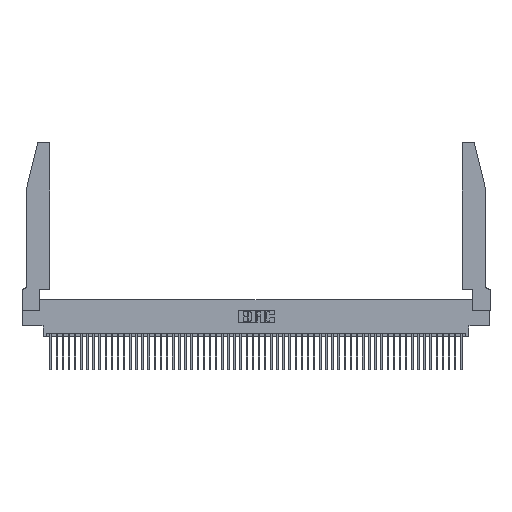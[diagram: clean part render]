
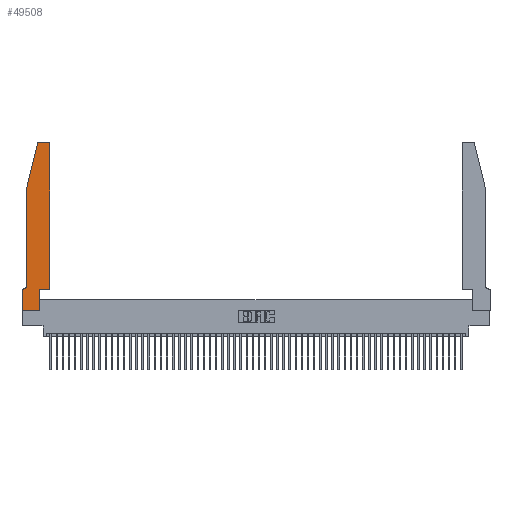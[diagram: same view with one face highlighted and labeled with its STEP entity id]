
A CAD part, top view. The second image highlights one B-rep face of the part: STEP entity #49508.
In plain terms, the highlighted planar face has unit normal (0, 0, 1).
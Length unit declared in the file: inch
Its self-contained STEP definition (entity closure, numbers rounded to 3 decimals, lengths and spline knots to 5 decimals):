
#418 = DIRECTION ( 'NONE',  ( 1., 0., 0. ) ) ;
#775 = EDGE_CURVE ( 'NONE', #7307, #12237, #3849, .T. ) ;
#871 = AXIS2_PLACEMENT_3D ( 'NONE', #14094, #43583, #18420 ) ;
#1311 = DIRECTION ( 'NONE',  ( 1., 0., 0. ) ) ;
#1388 = EDGE_CURVE ( 'NONE', #29535, #44781, #18639, .T. ) ;
#1393 = ORIENTED_EDGE ( 'NONE', *, *, #41156, .T. ) ;
#1676 = CARTESIAN_POINT ( 'NONE',  ( 0.4205, 2.75, 0.37 ) ) ;
#2209 = CARTESIAN_POINT ( 'NONE',  ( 0.25487, 2.72718, 0.37 ) ) ;
#3660 = CARTESIAN_POINT ( 'NONE',  ( 0.0755, 2., 0.37 ) ) ;
#3849 = LINE ( 'NONE', #41785, #36506 ) ;
#4893 = CARTESIAN_POINT ( 'NONE',  ( 0.2605, 2.75, 0.37 ) ) ;
#6025 = FACE_OUTER_BOUND ( 'NONE', #29176, .T. ) ;
#6207 = CARTESIAN_POINT ( 'NONE',  ( 0.4505, 0.35, 0.37 ) ) ;
#6626 = VERTEX_POINT ( 'NONE', #47167 ) ;
#6795 = ORIENTED_EDGE ( 'NONE', *, *, #48943, .T. ) ;
#7307 = VERTEX_POINT ( 'NONE', #44047 ) ;
#7408 = ORIENTED_EDGE ( 'NONE', *, *, #50088, .T. ) ;
#8753 = DIRECTION ( 'NONE',  ( -1., 0., 0. ) ) ;
#8770 = DIRECTION ( 'NONE',  ( 0., -1., 0. ) ) ;
#10470 = EDGE_CURVE ( 'NONE', #6626, #29535, #52792, .T. ) ;
#12237 = VERTEX_POINT ( 'NONE', #25831 ) ;
#12393 = VERTEX_POINT ( 'NONE', #30925 ) ;
#12711 = DIRECTION ( 'NONE',  ( 1., 0., 0. ) ) ;
#13014 = DIRECTION ( 'NONE',  ( -0.239, -0.971, 0. ) ) ;
#14094 = CARTESIAN_POINT ( 'NONE',  ( 0., 0.35, 0.37 ) ) ;
#14241 = ORIENTED_EDGE ( 'NONE', *, *, #775, .T. ) ;
#14365 = LINE ( 'NONE', #3660, #27088 ) ;
#14387 = LINE ( 'NONE', #29685, #36883 ) ;
#14700 = EDGE_CURVE ( 'NONE', #30006, #12393, #19690, .T. ) ;
#15366 = EDGE_CURVE ( 'NONE', #50289, #6626, #39972, .T. ) ;
#16240 = ORIENTED_EDGE ( 'NONE', *, *, #10470, .T. ) ;
#16377 = VERTEX_POINT ( 'NONE', #40725 ) ;
#17351 = CARTESIAN_POINT ( 'NONE',  ( 0.0755, 2., 0.37 ) ) ;
#17353 = CARTESIAN_POINT ( 'NONE',  ( 0.284, 2.75, 0.37 ) ) ;
#17538 = ORIENTED_EDGE ( 'NONE', *, *, #36465, .T. ) ;
#17938 = DIRECTION ( 'NONE',  ( -1., 0., 0. ) ) ;
#18100 = DIRECTION ( 'NONE',  ( 0., 1., 0. ) ) ;
#18420 = DIRECTION ( 'NONE',  ( 1., 0., 0. ) ) ;
#18639 = LINE ( 'NONE', #42083, #39715 ) ;
#19247 = CARTESIAN_POINT ( 'NONE',  ( 0., 0.35, 0.37 ) ) ;
#19675 = CIRCLE ( 'NONE', #27865, 0.03 ) ;
#19690 = LINE ( 'NONE', #17351, #28341 ) ;
#20626 = VERTEX_POINT ( 'NONE', #27876 ) ;
#23301 = CARTESIAN_POINT ( 'NONE',  ( 0., 0., 0.37 ) ) ;
#23875 = AXIS2_PLACEMENT_3D ( 'NONE', #50057, #25128, #54275 ) ;
#24315 = VECTOR ( 'NONE', #31812, 39.37008 ) ;
#25128 = DIRECTION ( 'NONE',  ( 0., 0., -1. ) ) ;
#25769 = AXIS2_PLACEMENT_3D ( 'NONE', #51171, #26213, #418 ) ;
#25831 = CARTESIAN_POINT ( 'NONE',  ( 0.4505, 0.35, 0.37 ) ) ;
#25879 = CARTESIAN_POINT ( 'NONE',  ( 0.0755, 0.35, 0.37 ) ) ;
#26213 = DIRECTION ( 'NONE',  ( 0., 0., 1. ) ) ;
#26536 = VECTOR ( 'NONE', #17938, 39.37008 ) ;
#27079 = DIRECTION ( 'NONE',  ( 0., 0., 1. ) ) ;
#27088 = VECTOR ( 'NONE', #8770, 39.37008 ) ;
#27865 = AXIS2_PLACEMENT_3D ( 'NONE', #52033, #27079, #1311 ) ;
#27876 = CARTESIAN_POINT ( 'NONE',  ( 0.4505, 2.72, 0.37 ) ) ;
#28341 = VECTOR ( 'NONE', #13014, 39.37008 ) ;
#29176 = EDGE_LOOP ( 'NONE', ( #17538, #7408, #34075, #32137, #33447, #16240, #31519, #53668, #1393, #14241, #6795, #33509 ) ) ;
#29295 = VECTOR ( 'NONE', #18100, 39.37008 ) ;
#29402 = EDGE_CURVE ( 'NONE', #20626, #43248, #19675, .T. ) ;
#29535 = VERTEX_POINT ( 'NONE', #19247 ) ;
#29685 = CARTESIAN_POINT ( 'NONE',  ( 0., 0., 0.37 ) ) ;
#30006 = VERTEX_POINT ( 'NONE', #2209 ) ;
#30714 = CARTESIAN_POINT ( 'NONE',  ( 0.2865, 0.35, 0.37 ) ) ;
#30925 = CARTESIAN_POINT ( 'NONE',  ( 0.0755, 2., 0.37 ) ) ;
#31519 = ORIENTED_EDGE ( 'NONE', *, *, #1388, .T. ) ;
#31544 = VERTEX_POINT ( 'NONE', #17353 ) ;
#31812 = DIRECTION ( 'NONE',  ( 0., 1., 0. ) ) ;
#32137 = ORIENTED_EDGE ( 'NONE', *, *, #37608, .T. ) ;
#33447 = ORIENTED_EDGE ( 'NONE', *, *, #15366, .T. ) ;
#33509 = ORIENTED_EDGE ( 'NONE', *, *, #29402, .T. ) ;
#34075 = ORIENTED_EDGE ( 'NONE', *, *, #14700, .T. ) ;
#34929 = EDGE_CURVE ( 'NONE', #44781, #16377, #14387, .T. ) ;
#35225 = PLANE ( 'NONE',  #871 ) ;
#35689 = CARTESIAN_POINT ( 'NONE',  ( 0.0755, 0.42, 0.37 ) ) ;
#36465 = EDGE_CURVE ( 'NONE', #43248, #31544, #37629, .T. ) ;
#36506 = VECTOR ( 'NONE', #45945, 39.37008 ) ;
#36717 = LINE ( 'NONE', #6207, #24315 ) ;
#36883 = VECTOR ( 'NONE', #12711, 39.37008 ) ;
#37608 = EDGE_CURVE ( 'NONE', #12393, #50289, #14365, .T. ) ;
#37629 = LINE ( 'NONE', #4893, #26536 ) ;
#37878 = DIRECTION ( 'NONE',  ( 0., -1., 0. ) ) ;
#39715 = VECTOR ( 'NONE', #37878, 39.37008 ) ;
#39972 = CIRCLE ( 'NONE', #23875, 0.07 ) ;
#40374 = LINE ( 'NONE', #30714, #29295 ) ;
#40725 = CARTESIAN_POINT ( 'NONE',  ( 0.2865, 0., 0.37 ) ) ;
#41156 = EDGE_CURVE ( 'NONE', #16377, #7307, #40374, .T. ) ;
#41721 = VECTOR ( 'NONE', #8753, 39.37008 ) ;
#41785 = CARTESIAN_POINT ( 'NONE',  ( 0.4505, 0.35, 0.37 ) ) ;
#42083 = CARTESIAN_POINT ( 'NONE',  ( 0., 0., 0.37 ) ) ;
#43248 = VERTEX_POINT ( 'NONE', #1676 ) ;
#43583 = DIRECTION ( 'NONE',  ( 0., 0., 1. ) ) ;
#44047 = CARTESIAN_POINT ( 'NONE',  ( 0.2865, 0.35, 0.37 ) ) ;
#44386 = CIRCLE ( 'NONE', #25769, 0.03 ) ;
#44781 = VERTEX_POINT ( 'NONE', #23301 ) ;
#45945 = DIRECTION ( 'NONE',  ( 1., 0., 0. ) ) ;
#47167 = CARTESIAN_POINT ( 'NONE',  ( 0.0055, 0.35, 0.37 ) ) ;
#48943 = EDGE_CURVE ( 'NONE', #12237, #20626, #36717, .T. ) ;
#49508 = ADVANCED_FACE ( 'NONE', ( #6025 ), #35225, .T. ) ;
#50057 = CARTESIAN_POINT ( 'NONE',  ( 0.0055, 0.42, 0.37 ) ) ;
#50088 = EDGE_CURVE ( 'NONE', #31544, #30006, #44386, .T. ) ;
#50289 = VERTEX_POINT ( 'NONE', #35689 ) ;
#51171 = CARTESIAN_POINT ( 'NONE',  ( 0.284, 2.72, 0.37 ) ) ;
#52033 = CARTESIAN_POINT ( 'NONE',  ( 0.4205, 2.72, 0.37 ) ) ;
#52792 = LINE ( 'NONE', #25879, #41721 ) ;
#53668 = ORIENTED_EDGE ( 'NONE', *, *, #34929, .T. ) ;
#54275 = DIRECTION ( 'NONE',  ( -1., 0., 0. ) ) ;
